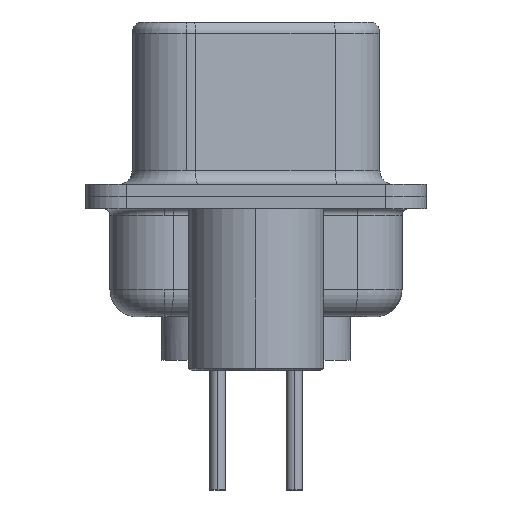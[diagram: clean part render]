
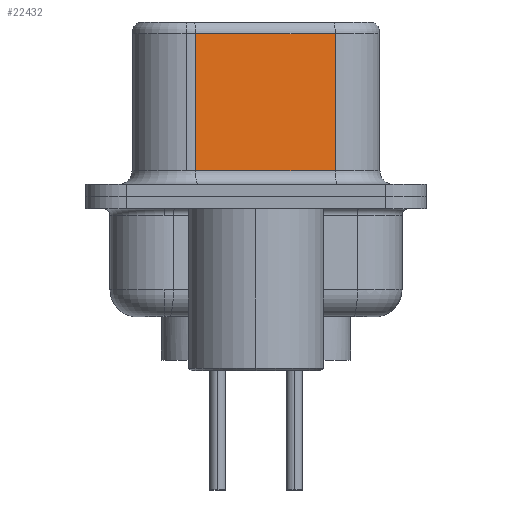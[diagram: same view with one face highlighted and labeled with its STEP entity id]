
A CAD part, left-side view. The second image highlights one B-rep face of the part: STEP entity #22432.
In plain terms, the highlighted planar face has unit normal (-0.985, -0.174, 0).
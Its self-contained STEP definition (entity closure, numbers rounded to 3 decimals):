
#723 = EDGE_LOOP ( 'NONE', ( #21602, #19837, #9092, #22001 ) ) ;
#834 = CARTESIAN_POINT ( 'NONE',  ( 4.58, -2.927, 6.02 ) ) ;
#1347 = VECTOR ( 'NONE', #23221, 1000. ) ;
#1842 = VERTEX_POINT ( 'NONE', #4005 ) ;
#2907 = DIRECTION ( 'NONE',  ( -0.174, 0.985, 0. ) ) ;
#3889 = VERTEX_POINT ( 'NONE', #11132 ) ;
#4005 = CARTESIAN_POINT ( 'NONE',  ( 4.58, -2.927, 0.95 ) ) ;
#5441 = EDGE_CURVE ( 'NONE', #16120, #1842, #5448, .T. ) ;
#5448 = LINE ( 'NONE', #6052, #22301 ) ;
#6052 = CARTESIAN_POINT ( 'NONE',  ( 4.58, -2.927, 0.95 ) ) ;
#7056 = CARTESIAN_POINT ( 'NONE',  ( 4.58, -2.927, 6.02 ) ) ;
#8064 = VECTOR ( 'NONE', #23879, 1000. ) ;
#9018 = DIRECTION ( 'NONE',  ( -0.174, 0.985, 0. ) ) ;
#9032 = PLANE ( 'NONE',  #22488 ) ;
#9092 = ORIENTED_EDGE ( 'NONE', *, *, #15073, .T. ) ;
#9470 = EDGE_CURVE ( 'NONE', #19008, #1842, #17995, .T. ) ;
#11132 = CARTESIAN_POINT ( 'NONE',  ( 3.67, 2.233, 6.02 ) ) ;
#12383 = CARTESIAN_POINT ( 'NONE',  ( 4.58, -2.927, 6.52 ) ) ;
#12813 = CARTESIAN_POINT ( 'NONE',  ( 4.58, -2.927, 6.52 ) ) ;
#14903 = DIRECTION ( 'NONE',  ( 0.985, 0.174, 0. ) ) ;
#15073 = EDGE_CURVE ( 'NONE', #3889, #16120, #17345, .T. ) ;
#15380 = LINE ( 'NONE', #7056, #23309 ) ;
#16120 = VERTEX_POINT ( 'NONE', #18144 ) ;
#17345 = LINE ( 'NONE', #25291, #1347 ) ;
#17995 = LINE ( 'NONE', #12383, #8064 ) ;
#18144 = CARTESIAN_POINT ( 'NONE',  ( 3.67, 2.233, 0.95 ) ) ;
#19008 = VERTEX_POINT ( 'NONE', #834 ) ;
#19192 = EDGE_CURVE ( 'NONE', #19008, #3889, #15380, .T. ) ;
#19837 = ORIENTED_EDGE ( 'NONE', *, *, #19192, .T. ) ;
#21602 = ORIENTED_EDGE ( 'NONE', *, *, #9470, .F. ) ;
#22001 = ORIENTED_EDGE ( 'NONE', *, *, #5441, .T. ) ;
#22301 = VECTOR ( 'NONE', #25728, 1000. ) ;
#22432 = ADVANCED_FACE ( 'NONE', ( #24821 ), #9032, .F. ) ;
#22488 = AXIS2_PLACEMENT_3D ( 'NONE', #12813, #14903, #2907 ) ;
#23221 = DIRECTION ( 'NONE',  ( 0., 0., -1. ) ) ;
#23309 = VECTOR ( 'NONE', #9018, 1000. ) ;
#23879 = DIRECTION ( 'NONE',  ( 0., 0., -1. ) ) ;
#24821 = FACE_OUTER_BOUND ( 'NONE', #723, .T. ) ;
#25291 = CARTESIAN_POINT ( 'NONE',  ( 3.67, 2.233, 6.52 ) ) ;
#25728 = DIRECTION ( 'NONE',  ( 0.174, -0.985, 0. ) ) ;
